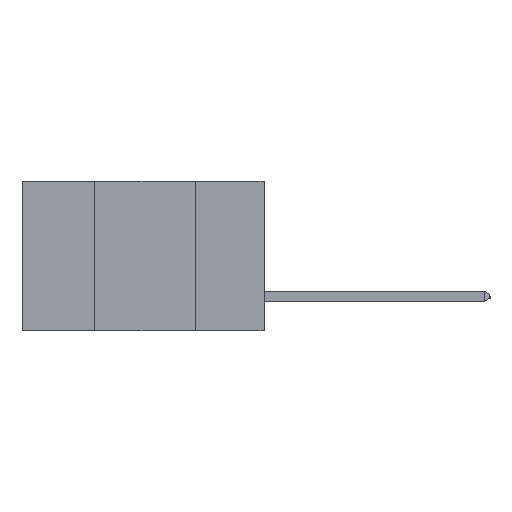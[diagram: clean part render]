
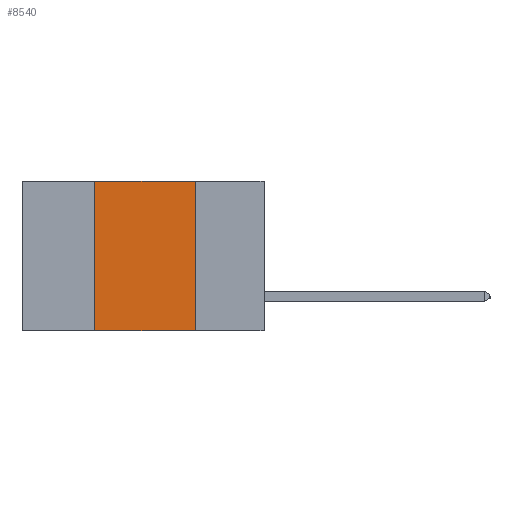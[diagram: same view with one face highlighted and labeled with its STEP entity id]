
A CAD part, left-side view. The second image highlights one B-rep face of the part: STEP entity #8540.
In plain terms, the highlighted planar face has unit normal (-1, 0, 0).
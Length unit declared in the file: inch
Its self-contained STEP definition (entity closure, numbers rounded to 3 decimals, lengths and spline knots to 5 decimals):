
#413 = VERTEX_POINT ( 'NONE', #10691 ) ;
#562 = CARTESIAN_POINT ( 'NONE',  ( 0., 0.6, 0. ) ) ;
#686 = CARTESIAN_POINT ( 'NONE',  ( 0., 0.17, 0. ) ) ;
#1399 = ORIENTED_EDGE ( 'NONE', *, *, #10623, .F. ) ;
#1681 = DIRECTION ( 'NONE',  ( 0., 0., -1. ) ) ;
#1908 = VERTEX_POINT ( 'NONE', #6128 ) ;
#2096 = LINE ( 'NONE', #5029, #4672 ) ;
#2360 = CARTESIAN_POINT ( 'NONE',  ( 0., 0.42, 0. ) ) ;
#2518 = ORIENTED_EDGE ( 'NONE', *, *, #11470, .F. ) ;
#2566 = CARTESIAN_POINT ( 'NONE',  ( 0., 0.6, 0. ) ) ;
#3831 = LINE ( 'NONE', #2566, #11862 ) ;
#4491 = ORIENTED_EDGE ( 'NONE', *, *, #7322, .T. ) ;
#4593 = DIRECTION ( 'NONE',  ( 0., 0., 1. ) ) ;
#4672 = VECTOR ( 'NONE', #7216, 39.37008 ) ;
#5029 = CARTESIAN_POINT ( 'NONE',  ( 0., 0.6, -0.37 ) ) ;
#5374 = VERTEX_POINT ( 'NONE', #7359 ) ;
#6128 = CARTESIAN_POINT ( 'NONE',  ( 0., 0.42, -0.37 ) ) ;
#6460 = VERTEX_POINT ( 'NONE', #10553 ) ;
#6934 = DIRECTION ( 'NONE',  ( 0., -1., 0. ) ) ;
#7090 = ORIENTED_EDGE ( 'NONE', *, *, #9427, .F. ) ;
#7137 = PLANE ( 'NONE',  #10848 ) ;
#7216 = DIRECTION ( 'NONE',  ( 0., -1., 0. ) ) ;
#7322 = EDGE_CURVE ( 'NONE', #1908, #5374, #2096, .T. ) ;
#7359 = CARTESIAN_POINT ( 'NONE',  ( 0., 0.17, -0.37 ) ) ;
#8173 = DIRECTION ( 'NONE',  ( 1., 0., 0. ) ) ;
#8540 = ADVANCED_FACE ( 'NONE', ( #8666 ), #7137, .F. ) ;
#8638 = LINE ( 'NONE', #2360, #11060 ) ;
#8666 = FACE_OUTER_BOUND ( 'NONE', #12033, .T. ) ;
#8989 = LINE ( 'NONE', #686, #12009 ) ;
#9427 = EDGE_CURVE ( 'NONE', #1908, #413, #8638, .T. ) ;
#10408 = DIRECTION ( 'NONE',  ( 0., 0., -1. ) ) ;
#10553 = CARTESIAN_POINT ( 'NONE',  ( 0., 0.17, 0. ) ) ;
#10623 = EDGE_CURVE ( 'NONE', #413, #6460, #3831, .T. ) ;
#10691 = CARTESIAN_POINT ( 'NONE',  ( 0., 0.42, 0. ) ) ;
#10848 = AXIS2_PLACEMENT_3D ( 'NONE', #562, #8173, #1681 ) ;
#11060 = VECTOR ( 'NONE', #4593, 39.37008 ) ;
#11470 = EDGE_CURVE ( 'NONE', #6460, #5374, #8989, .T. ) ;
#11862 = VECTOR ( 'NONE', #6934, 39.37008 ) ;
#12009 = VECTOR ( 'NONE', #10408, 39.37008 ) ;
#12033 = EDGE_LOOP ( 'NONE', ( #2518, #1399, #7090, #4491 ) ) ;
